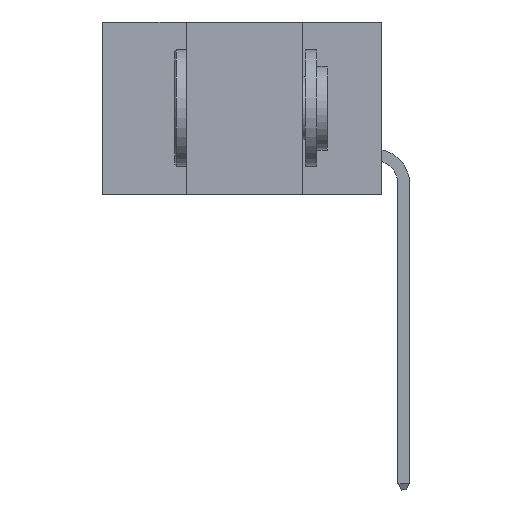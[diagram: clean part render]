
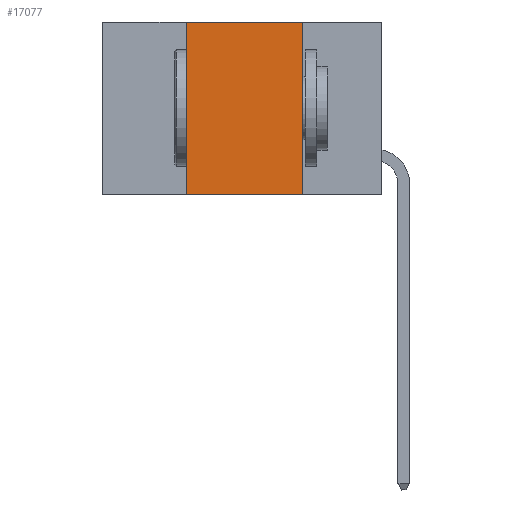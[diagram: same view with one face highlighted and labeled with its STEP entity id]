
A CAD part, left-side view. The second image highlights one B-rep face of the part: STEP entity #17077.
In plain terms, the highlighted planar face has unit normal (-1, 0, 0).
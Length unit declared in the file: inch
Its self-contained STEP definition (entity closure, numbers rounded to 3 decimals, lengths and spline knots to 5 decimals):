
#699 = FACE_OUTER_BOUND ( 'NONE', #1737, .T. ) ;
#1525 = VERTEX_POINT ( 'NONE', #7723 ) ;
#1737 = EDGE_LOOP ( 'NONE', ( #5452, #7981, #11249, #2382 ) ) ;
#2204 = DIRECTION ( 'NONE',  ( 0., 0., -1. ) ) ;
#2382 = ORIENTED_EDGE ( 'NONE', *, *, #9769, .T. ) ;
#3041 = CARTESIAN_POINT ( 'NONE',  ( 0., 0.42, 0. ) ) ;
#3191 = VERTEX_POINT ( 'NONE', #18474 ) ;
#4166 = CARTESIAN_POINT ( 'NONE',  ( 0., 0.6, 0. ) ) ;
#4272 = CARTESIAN_POINT ( 'NONE',  ( 0., 0.42, 0. ) ) ;
#4506 = LINE ( 'NONE', #5118, #22257 ) ;
#5118 = CARTESIAN_POINT ( 'NONE',  ( 0., 0.6, -0.37 ) ) ;
#5262 = DIRECTION ( 'NONE',  ( 1., 0., 0. ) ) ;
#5452 = ORIENTED_EDGE ( 'NONE', *, *, #16751, .F. ) ;
#7193 = DIRECTION ( 'NONE',  ( 0., 0., -1. ) ) ;
#7325 = VERTEX_POINT ( 'NONE', #4272 ) ;
#7723 = CARTESIAN_POINT ( 'NONE',  ( 0., 0.17, 0. ) ) ;
#7981 = ORIENTED_EDGE ( 'NONE', *, *, #13168, .F. ) ;
#9344 = PLANE ( 'NONE',  #10044 ) ;
#9769 = EDGE_CURVE ( 'NONE', #19537, #3191, #4506, .T. ) ;
#9927 = LINE ( 'NONE', #4166, #22906 ) ;
#10044 = AXIS2_PLACEMENT_3D ( 'NONE', #16873, #5262, #7193 ) ;
#11249 = ORIENTED_EDGE ( 'NONE', *, *, #22547, .F. ) ;
#12975 = LINE ( 'NONE', #3041, #22725 ) ;
#13168 = EDGE_CURVE ( 'NONE', #7325, #1525, #9927, .T. ) ;
#14107 = CARTESIAN_POINT ( 'NONE',  ( 0., 0.42, -0.37 ) ) ;
#15969 = DIRECTION ( 'NONE',  ( 0., 0., 1. ) ) ;
#16751 = EDGE_CURVE ( 'NONE', #1525, #3191, #21150, .T. ) ;
#16873 = CARTESIAN_POINT ( 'NONE',  ( 0., 0.6, 0. ) ) ;
#17077 = ADVANCED_FACE ( 'NONE', ( #699 ), #9344, .F. ) ;
#17272 = VECTOR ( 'NONE', #2204, 39.37008 ) ;
#17365 = DIRECTION ( 'NONE',  ( 0., -1., 0. ) ) ;
#18474 = CARTESIAN_POINT ( 'NONE',  ( 0., 0.17, -0.37 ) ) ;
#19537 = VERTEX_POINT ( 'NONE', #14107 ) ;
#20281 = DIRECTION ( 'NONE',  ( 0., -1., 0. ) ) ;
#20772 = CARTESIAN_POINT ( 'NONE',  ( 0., 0.17, 0. ) ) ;
#21150 = LINE ( 'NONE', #20772, #17272 ) ;
#22257 = VECTOR ( 'NONE', #20281, 39.37008 ) ;
#22547 = EDGE_CURVE ( 'NONE', #19537, #7325, #12975, .T. ) ;
#22725 = VECTOR ( 'NONE', #15969, 39.37008 ) ;
#22906 = VECTOR ( 'NONE', #17365, 39.37008 ) ;
